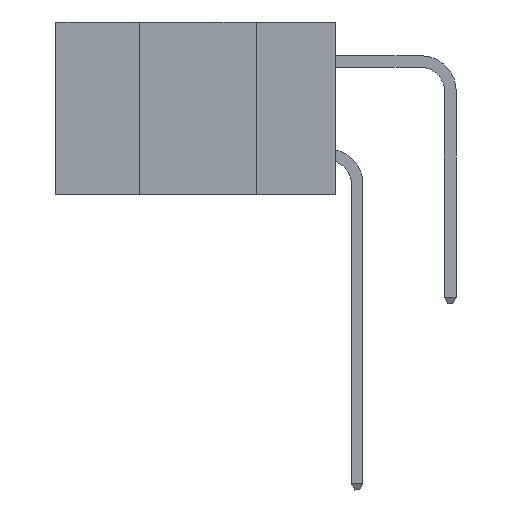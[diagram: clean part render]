
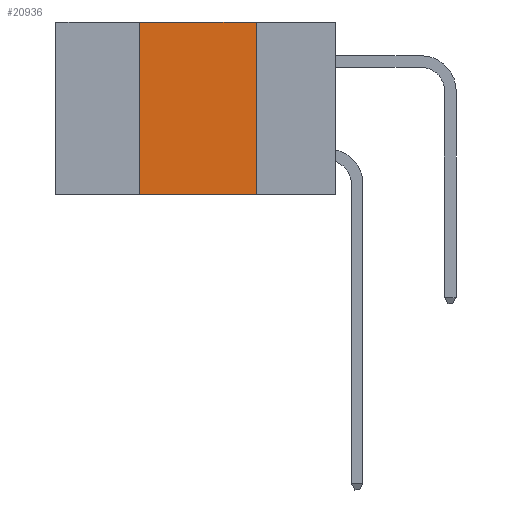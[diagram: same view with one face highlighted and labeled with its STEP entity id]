
A CAD part, left-side view. The second image highlights one B-rep face of the part: STEP entity #20936.
In plain terms, the highlighted planar face has unit normal (-1, 0, 0).
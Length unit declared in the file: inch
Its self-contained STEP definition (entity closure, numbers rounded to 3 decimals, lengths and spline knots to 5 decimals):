
#351 = LINE ( 'NONE', #8165, #19968 ) ;
#561 = LINE ( 'NONE', #13429, #1763 ) ;
#608 = EDGE_CURVE ( 'NONE', #23832, #12791, #6800, .T. ) ;
#1106 = CARTESIAN_POINT ( 'NONE',  ( 0., 0.6, 0. ) ) ;
#1763 = VECTOR ( 'NONE', #11690, 39.37008 ) ;
#2943 = FACE_OUTER_BOUND ( 'NONE', #6811, .T. ) ;
#3384 = CARTESIAN_POINT ( 'NONE',  ( 0., 0.42, 0. ) ) ;
#3415 = EDGE_CURVE ( 'NONE', #6715, #18113, #20358, .T. ) ;
#3829 = ORIENTED_EDGE ( 'NONE', *, *, #7006, .T. ) ;
#4968 = DIRECTION ( 'NONE',  ( 0., 0., -1. ) ) ;
#5458 = DIRECTION ( 'NONE',  ( 0., 0., 1. ) ) ;
#6715 = VERTEX_POINT ( 'NONE', #12573 ) ;
#6724 = DIRECTION ( 'NONE',  ( 0., 0., -1. ) ) ;
#6800 = LINE ( 'NONE', #21690, #13502 ) ;
#6811 = EDGE_LOOP ( 'NONE', ( #20220, #7626, #23951, #3829 ) ) ;
#7006 = EDGE_CURVE ( 'NONE', #6715, #12791, #561, .T. ) ;
#7626 = ORIENTED_EDGE ( 'NONE', *, *, #21186, .F. ) ;
#8165 = CARTESIAN_POINT ( 'NONE',  ( 0., 0.6, 0. ) ) ;
#11690 = DIRECTION ( 'NONE',  ( 0., -1., 0. ) ) ;
#12573 = CARTESIAN_POINT ( 'NONE',  ( 0., 0.42, -0.37 ) ) ;
#12791 = VERTEX_POINT ( 'NONE', #13441 ) ;
#13429 = CARTESIAN_POINT ( 'NONE',  ( 0., 0.6, -0.37 ) ) ;
#13441 = CARTESIAN_POINT ( 'NONE',  ( 0., 0.17, -0.37 ) ) ;
#13502 = VECTOR ( 'NONE', #4968, 39.37008 ) ;
#15156 = DIRECTION ( 'NONE',  ( 0., -1., 0. ) ) ;
#16011 = DIRECTION ( 'NONE',  ( 1., 0., 0. ) ) ;
#17836 = PLANE ( 'NONE',  #19175 ) ;
#17856 = CARTESIAN_POINT ( 'NONE',  ( 0., 0.17, 0. ) ) ;
#18113 = VERTEX_POINT ( 'NONE', #21696 ) ;
#19175 = AXIS2_PLACEMENT_3D ( 'NONE', #1106, #16011, #6724 ) ;
#19968 = VECTOR ( 'NONE', #15156, 39.37008 ) ;
#20220 = ORIENTED_EDGE ( 'NONE', *, *, #608, .F. ) ;
#20358 = LINE ( 'NONE', #3384, #22414 ) ;
#20936 = ADVANCED_FACE ( 'NONE', ( #2943 ), #17836, .F. ) ;
#21186 = EDGE_CURVE ( 'NONE', #18113, #23832, #351, .T. ) ;
#21690 = CARTESIAN_POINT ( 'NONE',  ( 0., 0.17, 0. ) ) ;
#21696 = CARTESIAN_POINT ( 'NONE',  ( 0., 0.42, 0. ) ) ;
#22414 = VECTOR ( 'NONE', #5458, 39.37008 ) ;
#23832 = VERTEX_POINT ( 'NONE', #17856 ) ;
#23951 = ORIENTED_EDGE ( 'NONE', *, *, #3415, .F. ) ;
